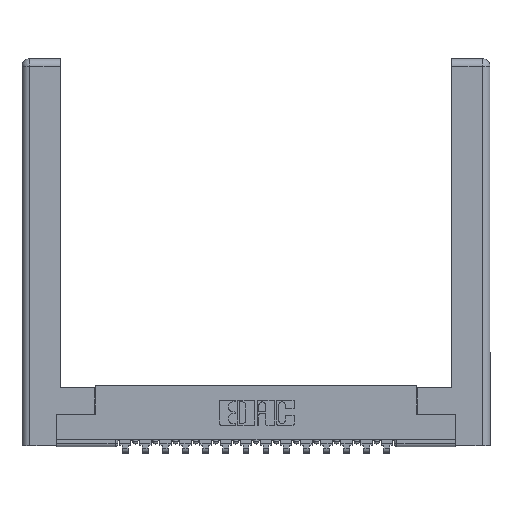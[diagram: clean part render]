
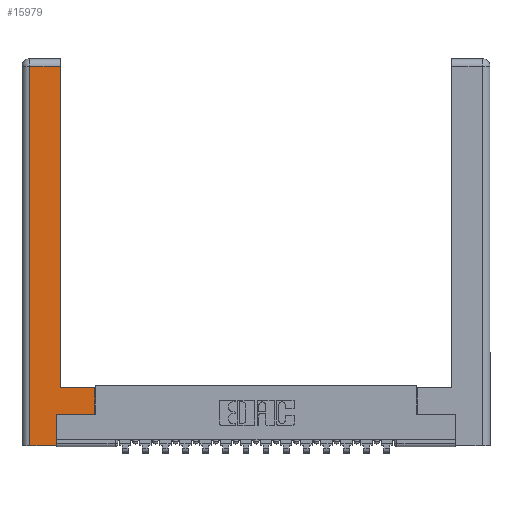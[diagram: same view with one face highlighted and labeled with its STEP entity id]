
A CAD part, top view. The second image highlights one B-rep face of the part: STEP entity #15979.
In plain terms, the highlighted planar face has unit normal (0, 0, 1).
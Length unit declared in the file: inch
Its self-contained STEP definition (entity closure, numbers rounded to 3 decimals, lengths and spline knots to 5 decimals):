
#45 = CARTESIAN_POINT ( 'NONE',  ( 0.565, 0.245, 0. ) ) ;
#157 = AXIS2_PLACEMENT_3D ( 'NONE', #7651, #10350, #1443 ) ;
#386 = LINE ( 'NONE', #16409, #15154 ) ;
#919 = ORIENTED_EDGE ( 'NONE', *, *, #9192, .T. ) ;
#943 = CARTESIAN_POINT ( 'NONE',  ( 0.295, 3., 0. ) ) ;
#1443 = DIRECTION ( 'NONE',  ( -1., 0., 0. ) ) ;
#1705 = EDGE_CURVE ( 'NONE', #12851, #8816, #14812, .T. ) ;
#2469 = ORIENTED_EDGE ( 'NONE', *, *, #15625, .T. ) ;
#2637 = VECTOR ( 'NONE', #12469, 39.37008 ) ;
#3027 = DIRECTION ( 'NONE',  ( -1., 0., 0. ) ) ;
#3066 = VERTEX_POINT ( 'NONE', #18106 ) ;
#3332 = DIRECTION ( 'NONE',  ( 1., 0., 0. ) ) ;
#3397 = CARTESIAN_POINT ( 'NONE',  ( 0.0615, 2.94, 0. ) ) ;
#3752 = LINE ( 'NONE', #18503, #2637 ) ;
#3882 = ORIENTED_EDGE ( 'NONE', *, *, #14815, .T. ) ;
#4286 = LINE ( 'NONE', #5716, #8753 ) ;
#4298 = ORIENTED_EDGE ( 'NONE', *, *, #13684, .T. ) ;
#4500 = FACE_OUTER_BOUND ( 'NONE', #5688, .T. ) ;
#4523 = CARTESIAN_POINT ( 'NONE',  ( 0.265, 0., 0. ) ) ;
#4762 = ORIENTED_EDGE ( 'NONE', *, *, #16057, .T. ) ;
#4798 = CARTESIAN_POINT ( 'NONE',  ( 0.295, 2.94, 0. ) ) ;
#4888 = ORIENTED_EDGE ( 'NONE', *, *, #15318, .T. ) ;
#4936 = VECTOR ( 'NONE', #17155, 39.37008 ) ;
#5518 = VERTEX_POINT ( 'NONE', #7035 ) ;
#5688 = EDGE_LOOP ( 'NONE', ( #919, #9978, #4888, #14241, #4298, #4762, #2469, #3882 ) ) ;
#5716 = CARTESIAN_POINT ( 'NONE',  ( 0.295, 0.45, 0. ) ) ;
#5753 = CARTESIAN_POINT ( 'NONE',  ( 0.0615, 2.94, 0. ) ) ;
#6324 = VECTOR ( 'NONE', #9330, 39.37008 ) ;
#6453 = CARTESIAN_POINT ( 'NONE',  ( 0.295, 0.45, 0. ) ) ;
#7035 = CARTESIAN_POINT ( 'NONE',  ( 0.265, 0., 0. ) ) ;
#7651 = CARTESIAN_POINT ( 'NONE',  ( 0., 0., 0. ) ) ;
#8753 = VECTOR ( 'NONE', #3027, 39.37008 ) ;
#8816 = VERTEX_POINT ( 'NONE', #5753 ) ;
#9192 = EDGE_CURVE ( 'NONE', #10747, #12851, #12626, .T. ) ;
#9330 = DIRECTION ( 'NONE',  ( -1., 0., 0. ) ) ;
#9978 = ORIENTED_EDGE ( 'NONE', *, *, #1705, .T. ) ;
#10000 = VECTOR ( 'NONE', #14772, 39.37008 ) ;
#10237 = VECTOR ( 'NONE', #13551, 39.37008 ) ;
#10350 = DIRECTION ( 'NONE',  ( 0., 0., -1. ) ) ;
#10484 = CARTESIAN_POINT ( 'NONE',  ( 0.265, 0.245, 0. ) ) ;
#10747 = VERTEX_POINT ( 'NONE', #6453 ) ;
#12277 = LINE ( 'NONE', #10484, #10237 ) ;
#12469 = DIRECTION ( 'NONE',  ( 0., -1., 0. ) ) ;
#12626 = LINE ( 'NONE', #943, #4936 ) ;
#12751 = VERTEX_POINT ( 'NONE', #14399 ) ;
#12851 = VERTEX_POINT ( 'NONE', #4798 ) ;
#13328 = DIRECTION ( 'NONE',  ( 0., 1., 0. ) ) ;
#13551 = DIRECTION ( 'NONE',  ( 0., 1., 0. ) ) ;
#13684 = EDGE_CURVE ( 'NONE', #5518, #15422, #12277, .T. ) ;
#13949 = VECTOR ( 'NONE', #3332, 39.37008 ) ;
#14241 = ORIENTED_EDGE ( 'NONE', *, *, #16876, .T. ) ;
#14399 = CARTESIAN_POINT ( 'NONE',  ( 0.0615, 0., 0. ) ) ;
#14772 = DIRECTION ( 'NONE',  ( 1., 0., 0. ) ) ;
#14812 = LINE ( 'NONE', #3397, #6324 ) ;
#14815 = EDGE_CURVE ( 'NONE', #3066, #10747, #4286, .T. ) ;
#15154 = VECTOR ( 'NONE', #13328, 39.37008 ) ;
#15318 = EDGE_CURVE ( 'NONE', #8816, #12751, #3752, .T. ) ;
#15422 = VERTEX_POINT ( 'NONE', #18131 ) ;
#15625 = EDGE_CURVE ( 'NONE', #18373, #3066, #386, .T. ) ;
#15979 = ADVANCED_FACE ( 'NONE', ( #4500 ), #16200, .F. ) ;
#16057 = EDGE_CURVE ( 'NONE', #15422, #18373, #16389, .T. ) ;
#16200 = PLANE ( 'NONE',  #157 ) ;
#16389 = LINE ( 'NONE', #16479, #13949 ) ;
#16409 = CARTESIAN_POINT ( 'NONE',  ( 0.565, 0.45, 0. ) ) ;
#16479 = CARTESIAN_POINT ( 'NONE',  ( 0.565, 0.245, 0. ) ) ;
#16876 = EDGE_CURVE ( 'NONE', #12751, #5518, #17656, .T. ) ;
#17155 = DIRECTION ( 'NONE',  ( 0., 1., 0. ) ) ;
#17656 = LINE ( 'NONE', #4523, #10000 ) ;
#18106 = CARTESIAN_POINT ( 'NONE',  ( 0.565, 0.45, 0. ) ) ;
#18131 = CARTESIAN_POINT ( 'NONE',  ( 0.265, 0.245, 0. ) ) ;
#18373 = VERTEX_POINT ( 'NONE', #45 ) ;
#18503 = CARTESIAN_POINT ( 'NONE',  ( 0.0615, 0., 0. ) ) ;
